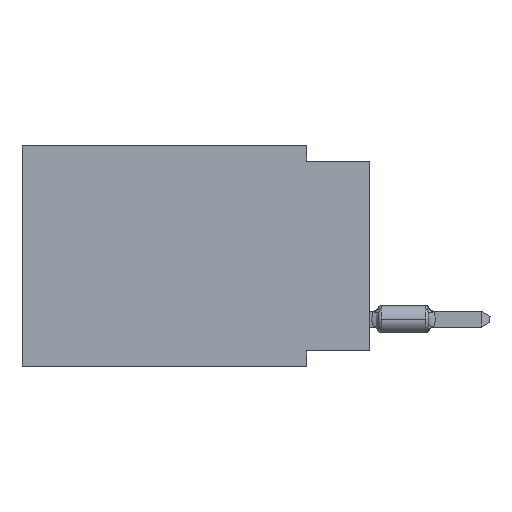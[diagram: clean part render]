
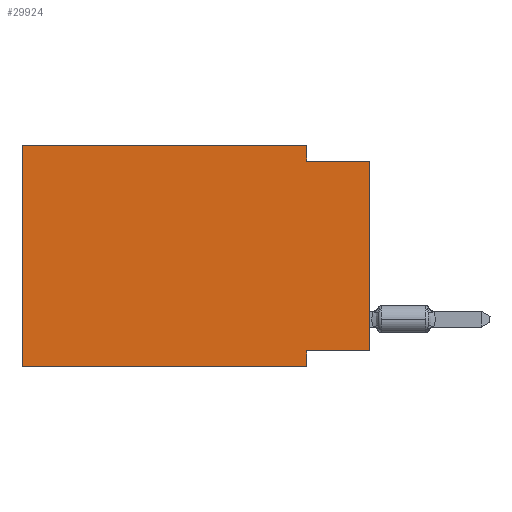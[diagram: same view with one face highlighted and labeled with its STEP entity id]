
A CAD part, left-side view. The second image highlights one B-rep face of the part: STEP entity #29924.
In plain terms, the highlighted planar face has unit normal (-1, 0, 0).
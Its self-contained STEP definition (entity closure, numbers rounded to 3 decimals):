
#165 = DIRECTION ( 'NONE',  ( 0., 0., -1. ) ) ;
#1107 = VERTEX_POINT ( 'NONE', #5086 ) ;
#1549 = CARTESIAN_POINT ( 'NONE',  ( 0., 2.54, -8.89 ) ) ;
#1663 = VERTEX_POINT ( 'NONE', #1549 ) ;
#2293 = CARTESIAN_POINT ( 'NONE',  ( 0., 0., -8.255 ) ) ;
#3273 = ORIENTED_EDGE ( 'NONE', *, *, #13403, .T. ) ;
#4005 = VERTEX_POINT ( 'NONE', #11602 ) ;
#4149 = ORIENTED_EDGE ( 'NONE', *, *, #23011, .F. ) ;
#5086 = CARTESIAN_POINT ( 'NONE',  ( 0., 2.54, -8.255 ) ) ;
#6785 = EDGE_CURVE ( 'NONE', #46793, #1663, #43476, .T. ) ;
#7176 = VERTEX_POINT ( 'NONE', #19430 ) ;
#7928 = DIRECTION ( 'NONE',  ( 0., 0., 1. ) ) ;
#8024 = DIRECTION ( 'NONE',  ( 0., -1., 0. ) ) ;
#8136 = ORIENTED_EDGE ( 'NONE', *, *, #18534, .F. ) ;
#8350 = CARTESIAN_POINT ( 'NONE',  ( 0., 13.97, 0. ) ) ;
#11075 = ORIENTED_EDGE ( 'NONE', *, *, #40941, .F. ) ;
#11602 = CARTESIAN_POINT ( 'NONE',  ( 0., 13.97, 0. ) ) ;
#11717 = CARTESIAN_POINT ( 'NONE',  ( 0., 13.97, 0. ) ) ;
#12614 = DIRECTION ( 'NONE',  ( 1., 0., 0. ) ) ;
#13137 = DIRECTION ( 'NONE',  ( 0., 0., -1. ) ) ;
#13403 = EDGE_CURVE ( 'NONE', #23792, #7176, #44417, .T. ) ;
#13745 = ORIENTED_EDGE ( 'NONE', *, *, #37798, .F. ) ;
#14244 = EDGE_CURVE ( 'NONE', #23792, #1107, #23840, .T. ) ;
#14316 = ORIENTED_EDGE ( 'NONE', *, *, #6785, .T. ) ;
#15168 = DIRECTION ( 'NONE',  ( 0., -1., 0. ) ) ;
#15858 = DIRECTION ( 'NONE',  ( 0., 1., 0. ) ) ;
#18482 = VECTOR ( 'NONE', #27949, 1000. ) ;
#18534 = EDGE_CURVE ( 'NONE', #46793, #4005, #24873, .T. ) ;
#18972 = AXIS2_PLACEMENT_3D ( 'NONE', #8350, #12614, #13137 ) ;
#19430 = CARTESIAN_POINT ( 'NONE',  ( 0., 0., -0.635 ) ) ;
#20600 = VERTEX_POINT ( 'NONE', #22605 ) ;
#20695 = CARTESIAN_POINT ( 'NONE',  ( 0., 0., 0. ) ) ;
#21523 = ORIENTED_EDGE ( 'NONE', *, *, #14244, .F. ) ;
#21827 = LINE ( 'NONE', #38063, #28501 ) ;
#22605 = CARTESIAN_POINT ( 'NONE',  ( 0., 2.54, -0.635 ) ) ;
#23011 = EDGE_CURVE ( 'NONE', #20600, #7176, #47391, .T. ) ;
#23226 = CARTESIAN_POINT ( 'NONE',  ( 0., 13.97, -8.89 ) ) ;
#23792 = VERTEX_POINT ( 'NONE', #2293 ) ;
#23840 = LINE ( 'NONE', #52335, #40084 ) ;
#23941 = LINE ( 'NONE', #11717, #18482 ) ;
#24461 = EDGE_LOOP ( 'NONE', ( #3273, #4149, #13745, #44170, #8136, #14316, #11075, #21523 ) ) ;
#24873 = LINE ( 'NONE', #45893, #26531 ) ;
#26531 = VECTOR ( 'NONE', #37373, 1000. ) ;
#27949 = DIRECTION ( 'NONE',  ( 0., -1., 0. ) ) ;
#28501 = VECTOR ( 'NONE', #29037, 1000. ) ;
#29037 = DIRECTION ( 'NONE',  ( 0., 0., -1. ) ) ;
#29112 = PLANE ( 'NONE',  #18972 ) ;
#29924 = ADVANCED_FACE ( 'NONE', ( #49351 ), #29112, .F. ) ;
#34944 = VERTEX_POINT ( 'NONE', #37308 ) ;
#35206 = EDGE_CURVE ( 'NONE', #4005, #34944, #23941, .T. ) ;
#36473 = VECTOR ( 'NONE', #165, 1000. ) ;
#36636 = CARTESIAN_POINT ( 'NONE',  ( 0., 2.54, -8.89 ) ) ;
#37308 = CARTESIAN_POINT ( 'NONE',  ( 0., 2.54, 0. ) ) ;
#37373 = DIRECTION ( 'NONE',  ( 0., 0., 1. ) ) ;
#37798 = EDGE_CURVE ( 'NONE', #34944, #20600, #21827, .T. ) ;
#38063 = CARTESIAN_POINT ( 'NONE',  ( 0., 2.54, 0. ) ) ;
#39998 = VECTOR ( 'NONE', #7928, 1000. ) ;
#40084 = VECTOR ( 'NONE', #15858, 1000. ) ;
#40114 = LINE ( 'NONE', #36636, #36473 ) ;
#40941 = EDGE_CURVE ( 'NONE', #1107, #1663, #40114, .T. ) ;
#42627 = CARTESIAN_POINT ( 'NONE',  ( 0., 0., -0.635 ) ) ;
#43338 = VECTOR ( 'NONE', #15168, 1000. ) ;
#43476 = LINE ( 'NONE', #23226, #49836 ) ;
#44170 = ORIENTED_EDGE ( 'NONE', *, *, #35206, .F. ) ;
#44417 = LINE ( 'NONE', #20695, #39998 ) ;
#45893 = CARTESIAN_POINT ( 'NONE',  ( 0., 13.97, 0. ) ) ;
#46793 = VERTEX_POINT ( 'NONE', #49074 ) ;
#47391 = LINE ( 'NONE', #42627, #43338 ) ;
#49074 = CARTESIAN_POINT ( 'NONE',  ( 0., 13.97, -8.89 ) ) ;
#49351 = FACE_OUTER_BOUND ( 'NONE', #24461, .T. ) ;
#49836 = VECTOR ( 'NONE', #8024, 1000. ) ;
#52335 = CARTESIAN_POINT ( 'NONE',  ( 0., 0., -8.255 ) ) ;
